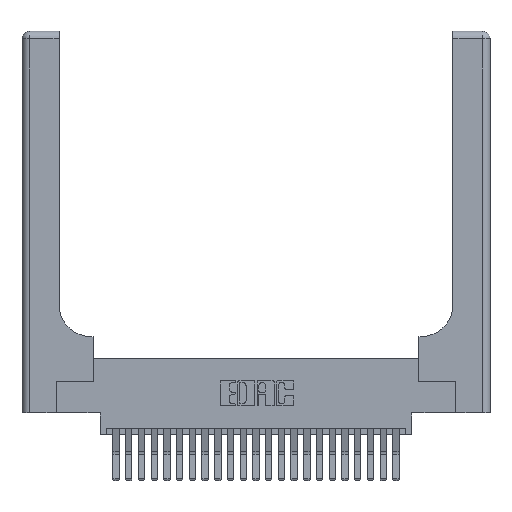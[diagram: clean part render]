
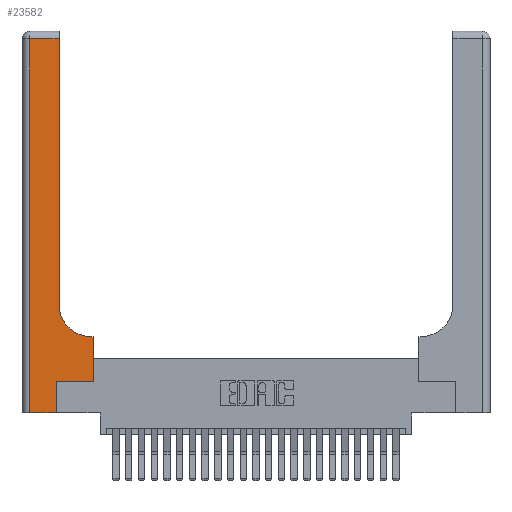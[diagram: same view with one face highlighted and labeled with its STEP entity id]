
A CAD part, top view. The second image highlights one B-rep face of the part: STEP entity #23582.
In plain terms, the highlighted planar face has unit normal (0, 0, 1).
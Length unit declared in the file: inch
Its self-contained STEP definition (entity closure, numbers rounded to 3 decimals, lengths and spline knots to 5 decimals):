
#1171 = VERTEX_POINT ( 'NONE', #7860 ) ;
#1587 = LINE ( 'NONE', #23486, #16996 ) ;
#1768 = ORIENTED_EDGE ( 'NONE', *, *, #13715, .T. ) ;
#1799 = LINE ( 'NONE', #7456, #17186 ) ;
#2312 = ORIENTED_EDGE ( 'NONE', *, *, #20564, .T. ) ;
#2807 = DIRECTION ( 'NONE',  ( -1., 0., 0. ) ) ;
#2808 = ORIENTED_EDGE ( 'NONE', *, *, #10833, .T. ) ;
#3109 = CARTESIAN_POINT ( 'NONE',  ( 0.2915, 3., 0.37 ) ) ;
#3757 = VECTOR ( 'NONE', #2807, 39.37008 ) ;
#3789 = CARTESIAN_POINT ( 'NONE',  ( 0.5415, 0.85, 0.37 ) ) ;
#4204 = VERTEX_POINT ( 'NONE', #4982 ) ;
#4716 = VERTEX_POINT ( 'NONE', #17644 ) ;
#4734 = EDGE_CURVE ( 'NONE', #4204, #25691, #14236, .T. ) ;
#4881 = CARTESIAN_POINT ( 'NONE',  ( 0., 3., 0.37 ) ) ;
#4981 = DIRECTION ( 'NONE',  ( 0., 0., -1. ) ) ;
#4982 = CARTESIAN_POINT ( 'NONE',  ( 0.5415, 0.6, 0.37 ) ) ;
#5017 = ORIENTED_EDGE ( 'NONE', *, *, #19250, .T. ) ;
#5153 = DIRECTION ( 'NONE',  ( 0., 1., 0. ) ) ;
#5304 = EDGE_CURVE ( 'NONE', #26035, #4204, #1587, .T. ) ;
#5801 = DIRECTION ( 'NONE',  ( 1., 0., 0. ) ) ;
#5839 = VECTOR ( 'NONE', #10435, 39.37008 ) ;
#6281 = CARTESIAN_POINT ( 'NONE',  ( 0.2915, 0.85, 0.37 ) ) ;
#6438 = VECTOR ( 'NONE', #23747, 39.37008 ) ;
#7180 = DIRECTION ( 'NONE',  ( 1., 0., 0. ) ) ;
#7456 = CARTESIAN_POINT ( 'NONE',  ( 0., 0., 0.37 ) ) ;
#7486 = CARTESIAN_POINT ( 'NONE',  ( 0.06, 3., 0.37 ) ) ;
#7860 = CARTESIAN_POINT ( 'NONE',  ( 0.06, 2.94, 0.37 ) ) ;
#8313 = LINE ( 'NONE', #3109, #18336 ) ;
#9087 = LINE ( 'NONE', #18867, #3757 ) ;
#9169 = EDGE_LOOP ( 'NONE', ( #1768, #20754, #20400, #2808, #5017, #2312, #20722, #22992, #21611 ) ) ;
#10320 = VERTEX_POINT ( 'NONE', #25169 ) ;
#10435 = DIRECTION ( 'NONE',  ( 0., 1., 0. ) ) ;
#10833 = EDGE_CURVE ( 'NONE', #14668, #10320, #1799, .T. ) ;
#11157 = CARTESIAN_POINT ( 'NONE',  ( 0.269, 0.25, 0.37 ) ) ;
#11209 = LINE ( 'NONE', #16370, #5839 ) ;
#11517 = DIRECTION ( 'NONE',  ( -1., 0., 0. ) ) ;
#11758 = CARTESIAN_POINT ( 'NONE',  ( 0.5585, 0.6, 0.37 ) ) ;
#11788 = CARTESIAN_POINT ( 'NONE',  ( 0.5585, 0.25, 0.37 ) ) ;
#11886 = CARTESIAN_POINT ( 'NONE',  ( 0.269, 0.25, 0.37 ) ) ;
#12735 = VECTOR ( 'NONE', #7180, 39.37008 ) ;
#12797 = EDGE_CURVE ( 'NONE', #16241, #26035, #17114, .T. ) ;
#13238 = VERTEX_POINT ( 'NONE', #11886 ) ;
#13544 = DIRECTION ( 'NONE',  ( 1., 0., 0. ) ) ;
#13570 = DIRECTION ( 'NONE',  ( 0., -1., 0. ) ) ;
#13715 = EDGE_CURVE ( 'NONE', #25691, #4716, #8313, .T. ) ;
#14236 = CIRCLE ( 'NONE', #17948, 0.25 ) ;
#14256 = CARTESIAN_POINT ( 'NONE',  ( 0.5585, 0.25, 0.37 ) ) ;
#14625 = LINE ( 'NONE', #11157, #12735 ) ;
#14668 = VERTEX_POINT ( 'NONE', #24226 ) ;
#16241 = VERTEX_POINT ( 'NONE', #14256 ) ;
#16370 = CARTESIAN_POINT ( 'NONE',  ( 0.269, 0., 0.37 ) ) ;
#16982 = PLANE ( 'NONE',  #25367 ) ;
#16996 = VECTOR ( 'NONE', #11517, 39.37008 ) ;
#17114 = LINE ( 'NONE', #11788, #6438 ) ;
#17186 = VECTOR ( 'NONE', #13544, 39.37008 ) ;
#17644 = CARTESIAN_POINT ( 'NONE',  ( 0.2915, 2.94, 0.37 ) ) ;
#17819 = DIRECTION ( 'NONE',  ( 0., 0., -1. ) ) ;
#17948 = AXIS2_PLACEMENT_3D ( 'NONE', #3789, #17819, #5801 ) ;
#18336 = VECTOR ( 'NONE', #5153, 39.37008 ) ;
#18867 = CARTESIAN_POINT ( 'NONE',  ( 0., 2.94, 0.37 ) ) ;
#18975 = DIRECTION ( 'NONE',  ( -1., 0., 0. ) ) ;
#19250 = EDGE_CURVE ( 'NONE', #10320, #13238, #11209, .T. ) ;
#20072 = LINE ( 'NONE', #7486, #24754 ) ;
#20400 = ORIENTED_EDGE ( 'NONE', *, *, #24690, .T. ) ;
#20564 = EDGE_CURVE ( 'NONE', #13238, #16241, #14625, .T. ) ;
#20722 = ORIENTED_EDGE ( 'NONE', *, *, #12797, .T. ) ;
#20754 = ORIENTED_EDGE ( 'NONE', *, *, #24501, .T. ) ;
#21611 = ORIENTED_EDGE ( 'NONE', *, *, #4734, .T. ) ;
#22992 = ORIENTED_EDGE ( 'NONE', *, *, #5304, .T. ) ;
#23486 = CARTESIAN_POINT ( 'NONE',  ( 0.2915, 0.6, 0.37 ) ) ;
#23582 = ADVANCED_FACE ( 'NONE', ( #24775 ), #16982, .F. ) ;
#23747 = DIRECTION ( 'NONE',  ( 0., 1., 0. ) ) ;
#24226 = CARTESIAN_POINT ( 'NONE',  ( 0.06, 0., 0.37 ) ) ;
#24501 = EDGE_CURVE ( 'NONE', #4716, #1171, #9087, .T. ) ;
#24690 = EDGE_CURVE ( 'NONE', #1171, #14668, #20072, .T. ) ;
#24754 = VECTOR ( 'NONE', #13570, 39.37008 ) ;
#24775 = FACE_OUTER_BOUND ( 'NONE', #9169, .T. ) ;
#25169 = CARTESIAN_POINT ( 'NONE',  ( 0.269, 0., 0.37 ) ) ;
#25367 = AXIS2_PLACEMENT_3D ( 'NONE', #4881, #4981, #18975 ) ;
#25691 = VERTEX_POINT ( 'NONE', #6281 ) ;
#26035 = VERTEX_POINT ( 'NONE', #11758 ) ;
